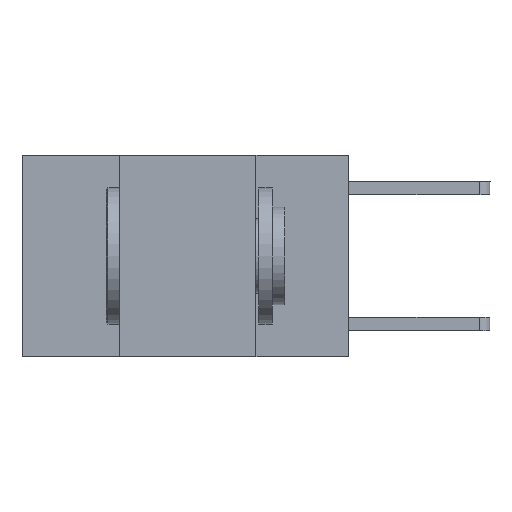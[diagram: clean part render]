
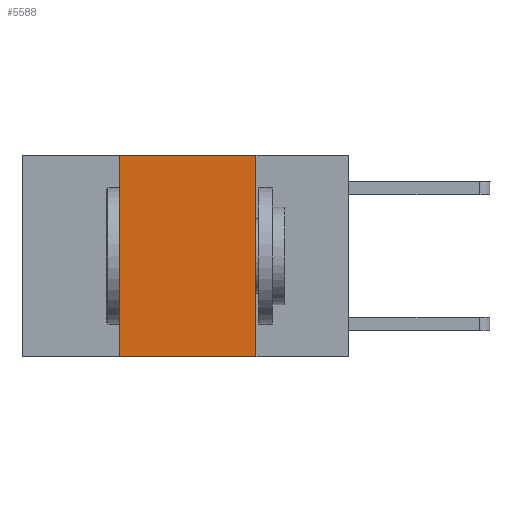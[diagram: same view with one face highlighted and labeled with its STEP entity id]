
A CAD part, left-side view. The second image highlights one B-rep face of the part: STEP entity #5588.
In plain terms, the highlighted planar face has unit normal (-1, 0, 0).
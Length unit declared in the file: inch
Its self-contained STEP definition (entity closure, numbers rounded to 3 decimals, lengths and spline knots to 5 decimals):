
#965 = VERTEX_POINT ( 'NONE', #5462 ) ;
#1074 = EDGE_CURVE ( 'NONE', #9282, #965, #6182, .T. ) ;
#1255 = FACE_OUTER_BOUND ( 'NONE', #4423, .T. ) ;
#1735 = ORIENTED_EDGE ( 'NONE', *, *, #2279, .T. ) ;
#1881 = DIRECTION ( 'NONE',  ( 0., -1., 0. ) ) ;
#2066 = VERTEX_POINT ( 'NONE', #8592 ) ;
#2233 = VECTOR ( 'NONE', #5165, 39.37008 ) ;
#2269 = LINE ( 'NONE', #5928, #2233 ) ;
#2279 = EDGE_CURVE ( 'NONE', #2066, #6914, #8442, .T. ) ;
#2282 = CARTESIAN_POINT ( 'NONE',  ( 0., 0.17, 0. ) ) ;
#2634 = AXIS2_PLACEMENT_3D ( 'NONE', #7180, #7137, #9192 ) ;
#3272 = ORIENTED_EDGE ( 'NONE', *, *, #1074, .F. ) ;
#3569 = VECTOR ( 'NONE', #1881, 39.37008 ) ;
#4423 = EDGE_LOOP ( 'NONE', ( #9172, #3272, #7362, #1735 ) ) ;
#4681 = VECTOR ( 'NONE', #6906, 39.37008 ) ;
#4787 = CARTESIAN_POINT ( 'NONE',  ( 0., 0.17, -0.37 ) ) ;
#5165 = DIRECTION ( 'NONE',  ( 0., 0., 1. ) ) ;
#5177 = DIRECTION ( 'NONE',  ( 0., 0., -1. ) ) ;
#5462 = CARTESIAN_POINT ( 'NONE',  ( 0., 0.17, 0. ) ) ;
#5588 = ADVANCED_FACE ( 'NONE', ( #1255 ), #6271, .F. ) ;
#5891 = LINE ( 'NONE', #2282, #7099 ) ;
#5928 = CARTESIAN_POINT ( 'NONE',  ( 0., 0.42, 0. ) ) ;
#6182 = LINE ( 'NONE', #8430, #3569 ) ;
#6271 = PLANE ( 'NONE',  #2634 ) ;
#6906 = DIRECTION ( 'NONE',  ( 0., -1., 0. ) ) ;
#6914 = VERTEX_POINT ( 'NONE', #4787 ) ;
#7099 = VECTOR ( 'NONE', #5177, 39.37008 ) ;
#7137 = DIRECTION ( 'NONE',  ( 1., 0., 0. ) ) ;
#7180 = CARTESIAN_POINT ( 'NONE',  ( 0., 0.6, 0. ) ) ;
#7334 = EDGE_CURVE ( 'NONE', #965, #6914, #5891, .T. ) ;
#7362 = ORIENTED_EDGE ( 'NONE', *, *, #7721, .F. ) ;
#7628 = CARTESIAN_POINT ( 'NONE',  ( 0., 0.6, -0.37 ) ) ;
#7721 = EDGE_CURVE ( 'NONE', #2066, #9282, #2269, .T. ) ;
#8430 = CARTESIAN_POINT ( 'NONE',  ( 0., 0.6, 0. ) ) ;
#8442 = LINE ( 'NONE', #7628, #4681 ) ;
#8592 = CARTESIAN_POINT ( 'NONE',  ( 0., 0.42, -0.37 ) ) ;
#9172 = ORIENTED_EDGE ( 'NONE', *, *, #7334, .F. ) ;
#9192 = DIRECTION ( 'NONE',  ( 0., 0., -1. ) ) ;
#9282 = VERTEX_POINT ( 'NONE', #9376 ) ;
#9376 = CARTESIAN_POINT ( 'NONE',  ( 0., 0.42, 0. ) ) ;
